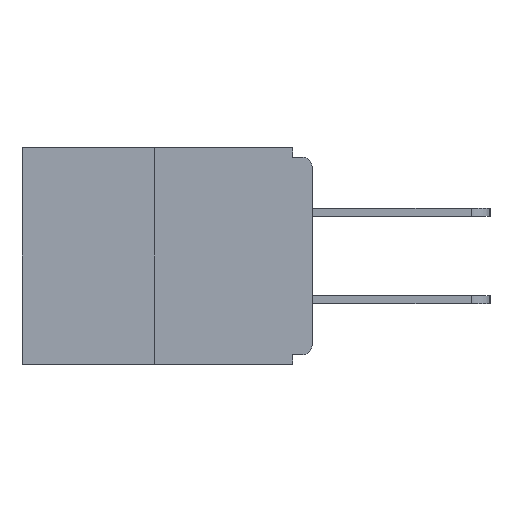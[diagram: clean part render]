
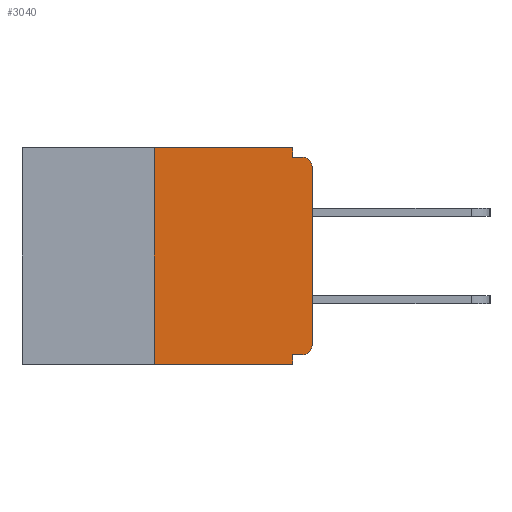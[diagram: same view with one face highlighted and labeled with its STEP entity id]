
A CAD part, left-side view. The second image highlights one B-rep face of the part: STEP entity #3040.
In plain terms, the highlighted planar face has unit normal (-1, 0, 0).
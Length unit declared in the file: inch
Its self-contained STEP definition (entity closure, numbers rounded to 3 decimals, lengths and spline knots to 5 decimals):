
#90 = VERTEX_POINT ( 'NONE', #21578 ) ;
#133 = VECTOR ( 'NONE', #4491, 39.37008 ) ;
#497 = VERTEX_POINT ( 'NONE', #9650 ) ;
#1239 = EDGE_CURVE ( 'NONE', #19500, #9385, #27447, .T. ) ;
#1266 = VERTEX_POINT ( 'NONE', #13787 ) ;
#2186 = VERTEX_POINT ( 'NONE', #7288 ) ;
#2366 = ORIENTED_EDGE ( 'NONE', *, *, #5089, .F. ) ;
#2691 = DIRECTION ( 'NONE',  ( 0., -1., 0. ) ) ;
#3040 = ADVANCED_FACE ( 'NONE', ( #15671 ), #23392, .F. ) ;
#3324 = CARTESIAN_POINT ( 'NONE',  ( 0., 0.25, -0.343 ) ) ;
#4178 = DIRECTION ( 'NONE',  ( 0., -1., 0. ) ) ;
#4491 = DIRECTION ( 'NONE',  ( 0., 0., 1. ) ) ;
#4695 = VERTEX_POINT ( 'NONE', #16260 ) ;
#5055 = LINE ( 'NONE', #23643, #20157 ) ;
#5057 = CARTESIAN_POINT ( 'NONE',  ( 0., 0.031, -0.343 ) ) ;
#5089 = EDGE_CURVE ( 'NONE', #16033, #1266, #9407, .T. ) ;
#5925 = ORIENTED_EDGE ( 'NONE', *, *, #27203, .F. ) ;
#5962 = VERTEX_POINT ( 'NONE', #28357 ) ;
#6979 = CARTESIAN_POINT ( 'NONE',  ( 0., 0.46, -0.343 ) ) ;
#6984 = CARTESIAN_POINT ( 'NONE',  ( 0., 0., -0.015 ) ) ;
#7288 = CARTESIAN_POINT ( 'NONE',  ( 0., 0.031, 0. ) ) ;
#8196 = VECTOR ( 'NONE', #24564, 39.37008 ) ;
#8279 = CARTESIAN_POINT ( 'NONE',  ( 0., 0.031, -0.015 ) ) ;
#8303 = DIRECTION ( 'NONE',  ( 0., 0., -1. ) ) ;
#8719 = ORIENTED_EDGE ( 'NONE', *, *, #14859, .T. ) ;
#9247 = CARTESIAN_POINT ( 'NONE',  ( 0., 0.015, -0.313 ) ) ;
#9385 = VERTEX_POINT ( 'NONE', #21032 ) ;
#9407 = LINE ( 'NONE', #17908, #133 ) ;
#9650 = CARTESIAN_POINT ( 'NONE',  ( 0., 0., -0.03 ) ) ;
#10219 = CARTESIAN_POINT ( 'NONE',  ( 0., 0.46, 0. ) ) ;
#10314 = ORIENTED_EDGE ( 'NONE', *, *, #22894, .T. ) ;
#10344 = AXIS2_PLACEMENT_3D ( 'NONE', #9247, #15737, #24795 ) ;
#10548 = VECTOR ( 'NONE', #27999, 39.37008 ) ;
#10557 = CARTESIAN_POINT ( 'NONE',  ( 0., 0.46, 0. ) ) ;
#10582 = AXIS2_PLACEMENT_3D ( 'NONE', #23993, #10815, #26756 ) ;
#10607 = CARTESIAN_POINT ( 'NONE',  ( 0., 0., -0.328 ) ) ;
#10696 = EDGE_CURVE ( 'NONE', #16033, #16487, #12461, .T. ) ;
#10759 = VECTOR ( 'NONE', #2691, 39.37008 ) ;
#10764 = EDGE_CURVE ( 'NONE', #1266, #2186, #27612, .T. ) ;
#10815 = DIRECTION ( 'NONE',  ( -1., 0., 0. ) ) ;
#11665 = ORIENTED_EDGE ( 'NONE', *, *, #10764, .F. ) ;
#12147 = DIRECTION ( 'NONE',  ( 0., 0., -1. ) ) ;
#12461 = LINE ( 'NONE', #6979, #10759 ) ;
#13577 = EDGE_LOOP ( 'NONE', ( #11665, #2366, #21054, #26506, #19954, #18524, #8719, #10314, #18030, #5925 ) ) ;
#13728 = CIRCLE ( 'NONE', #10582, 0.015 ) ;
#13787 = CARTESIAN_POINT ( 'NONE',  ( 0., 0.25, 0. ) ) ;
#14859 = EDGE_CURVE ( 'NONE', #90, #497, #5055, .T. ) ;
#15671 = FACE_OUTER_BOUND ( 'NONE', #13577, .T. ) ;
#15737 = DIRECTION ( 'NONE',  ( -1., 0., 0. ) ) ;
#16033 = VERTEX_POINT ( 'NONE', #3324 ) ;
#16260 = CARTESIAN_POINT ( 'NONE',  ( 0., 0.015, -0.328 ) ) ;
#16487 = VERTEX_POINT ( 'NONE', #19654 ) ;
#16832 = CARTESIAN_POINT ( 'NONE',  ( 0., 0.031, 0. ) ) ;
#17783 = LINE ( 'NONE', #10607, #10548 ) ;
#17908 = CARTESIAN_POINT ( 'NONE',  ( 0., 0.25, 0. ) ) ;
#18030 = ORIENTED_EDGE ( 'NONE', *, *, #1239, .F. ) ;
#18524 = ORIENTED_EDGE ( 'NONE', *, *, #27441, .T. ) ;
#19284 = AXIS2_PLACEMENT_3D ( 'NONE', #10219, #20899, #12147 ) ;
#19500 = VERTEX_POINT ( 'NONE', #8279 ) ;
#19654 = CARTESIAN_POINT ( 'NONE',  ( 0., 0.031, -0.343 ) ) ;
#19954 = ORIENTED_EDGE ( 'NONE', *, *, #24352, .F. ) ;
#20097 = VECTOR ( 'NONE', #8303, 39.37008 ) ;
#20157 = VECTOR ( 'NONE', #21530, 39.37008 ) ;
#20899 = DIRECTION ( 'NONE',  ( 1., 0., 0. ) ) ;
#21032 = CARTESIAN_POINT ( 'NONE',  ( 0., 0.015, -0.015 ) ) ;
#21054 = ORIENTED_EDGE ( 'NONE', *, *, #10696, .T. ) ;
#21530 = DIRECTION ( 'NONE',  ( 0., 0., 1. ) ) ;
#21578 = CARTESIAN_POINT ( 'NONE',  ( 0., 0., -0.313 ) ) ;
#22770 = DIRECTION ( 'NONE',  ( 0., 0., -1. ) ) ;
#22894 = EDGE_CURVE ( 'NONE', #497, #9385, #13728, .T. ) ;
#23141 = VECTOR ( 'NONE', #4178, 39.37008 ) ;
#23392 = PLANE ( 'NONE',  #19284 ) ;
#23520 = LINE ( 'NONE', #16832, #20097 ) ;
#23643 = CARTESIAN_POINT ( 'NONE',  ( 0., 0., 0. ) ) ;
#23993 = CARTESIAN_POINT ( 'NONE',  ( 0., 0.015, -0.03 ) ) ;
#24352 = EDGE_CURVE ( 'NONE', #4695, #5962, #17783, .T. ) ;
#24564 = DIRECTION ( 'NONE',  ( 0., -1., 0. ) ) ;
#24795 = DIRECTION ( 'NONE',  ( 0., 0., -1. ) ) ;
#25917 = CIRCLE ( 'NONE', #10344, 0.015 ) ;
#25975 = LINE ( 'NONE', #5057, #27687 ) ;
#26506 = ORIENTED_EDGE ( 'NONE', *, *, #26612, .F. ) ;
#26612 = EDGE_CURVE ( 'NONE', #5962, #16487, #25975, .T. ) ;
#26756 = DIRECTION ( 'NONE',  ( 0., 0., -1. ) ) ;
#27203 = EDGE_CURVE ( 'NONE', #2186, #19500, #23520, .T. ) ;
#27441 = EDGE_CURVE ( 'NONE', #4695, #90, #25917, .T. ) ;
#27447 = LINE ( 'NONE', #6984, #8196 ) ;
#27612 = LINE ( 'NONE', #10557, #23141 ) ;
#27687 = VECTOR ( 'NONE', #22770, 39.37008 ) ;
#27999 = DIRECTION ( 'NONE',  ( 0., 1., 0. ) ) ;
#28357 = CARTESIAN_POINT ( 'NONE',  ( 0., 0.031, -0.328 ) ) ;
